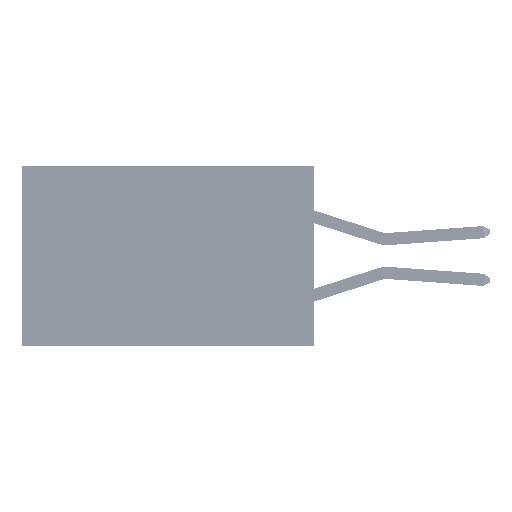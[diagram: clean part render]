
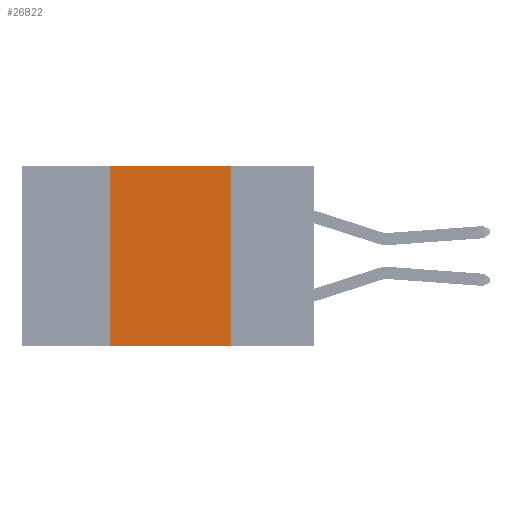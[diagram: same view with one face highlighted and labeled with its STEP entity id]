
A CAD part, left-side view. The second image highlights one B-rep face of the part: STEP entity #26822.
In plain terms, the highlighted planar face has unit normal (-1, 0, 0).
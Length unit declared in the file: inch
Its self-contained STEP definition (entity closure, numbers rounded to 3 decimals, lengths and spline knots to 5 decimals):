
#874 = LINE ( 'NONE', #43589, #41754 ) ;
#2781 = CARTESIAN_POINT ( 'NONE',  ( 0., 0.6, -0.37 ) ) ;
#5047 = EDGE_CURVE ( 'NONE', #17926, #50113, #16506, .T. ) ;
#11202 = CARTESIAN_POINT ( 'NONE',  ( 0., 0.17, 0. ) ) ;
#12636 = AXIS2_PLACEMENT_3D ( 'NONE', #21659, #36996, #25250 ) ;
#13988 = VECTOR ( 'NONE', #33858, 39.37008 ) ;
#16106 = LINE ( 'NONE', #38176, #18560 ) ;
#16506 = LINE ( 'NONE', #49232, #13988 ) ;
#17926 = VERTEX_POINT ( 'NONE', #30883 ) ;
#18411 = ORIENTED_EDGE ( 'NONE', *, *, #45184, .F. ) ;
#18560 = VECTOR ( 'NONE', #22290, 39.37008 ) ;
#18570 = DIRECTION ( 'NONE',  ( 0., -1., 0. ) ) ;
#19530 = VERTEX_POINT ( 'NONE', #41727 ) ;
#19703 = FACE_OUTER_BOUND ( 'NONE', #40536, .T. ) ;
#21659 = CARTESIAN_POINT ( 'NONE',  ( 0., 0.6, 0. ) ) ;
#22290 = DIRECTION ( 'NONE',  ( 0., -1., 0. ) ) ;
#23846 = CARTESIAN_POINT ( 'NONE',  ( 0., 0.42, 0. ) ) ;
#25250 = DIRECTION ( 'NONE',  ( 0., 0., -1. ) ) ;
#25424 = PLANE ( 'NONE',  #12636 ) ;
#26822 = ADVANCED_FACE ( 'NONE', ( #19703 ), #25424, .F. ) ;
#28569 = VECTOR ( 'NONE', #18570, 39.37008 ) ;
#30401 = EDGE_CURVE ( 'NONE', #50113, #42521, #16106, .T. ) ;
#30883 = CARTESIAN_POINT ( 'NONE',  ( 0., 0.42, -0.37 ) ) ;
#33858 = DIRECTION ( 'NONE',  ( 0., 0., 1. ) ) ;
#34397 = ORIENTED_EDGE ( 'NONE', *, *, #30401, .F. ) ;
#36996 = DIRECTION ( 'NONE',  ( 1., 0., 0. ) ) ;
#38176 = CARTESIAN_POINT ( 'NONE',  ( 0., 0.6, 0. ) ) ;
#40536 = EDGE_LOOP ( 'NONE', ( #18411, #34397, #48876, #47798 ) ) ;
#40944 = LINE ( 'NONE', #2781, #28569 ) ;
#41560 = EDGE_CURVE ( 'NONE', #17926, #19530, #40944, .T. ) ;
#41727 = CARTESIAN_POINT ( 'NONE',  ( 0., 0.17, -0.37 ) ) ;
#41754 = VECTOR ( 'NONE', #51239, 39.37008 ) ;
#42521 = VERTEX_POINT ( 'NONE', #11202 ) ;
#43589 = CARTESIAN_POINT ( 'NONE',  ( 0., 0.17, 0. ) ) ;
#45184 = EDGE_CURVE ( 'NONE', #42521, #19530, #874, .T. ) ;
#47798 = ORIENTED_EDGE ( 'NONE', *, *, #41560, .T. ) ;
#48876 = ORIENTED_EDGE ( 'NONE', *, *, #5047, .F. ) ;
#49232 = CARTESIAN_POINT ( 'NONE',  ( 0., 0.42, 0. ) ) ;
#50113 = VERTEX_POINT ( 'NONE', #23846 ) ;
#51239 = DIRECTION ( 'NONE',  ( 0., 0., -1. ) ) ;
